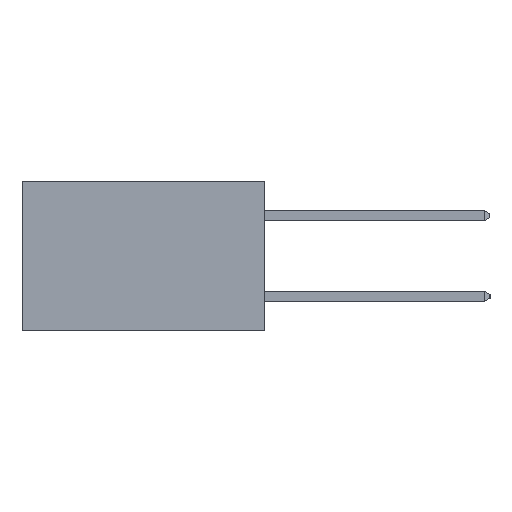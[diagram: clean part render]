
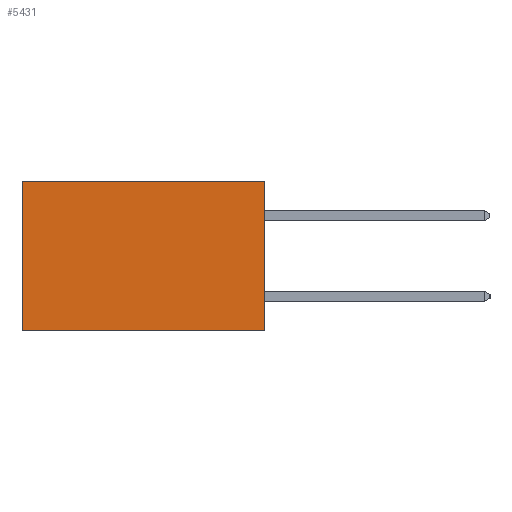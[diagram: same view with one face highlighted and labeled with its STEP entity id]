
A CAD part, left-side view. The second image highlights one B-rep face of the part: STEP entity #5431.
In plain terms, the highlighted planar face has unit normal (-1, 0, 0).
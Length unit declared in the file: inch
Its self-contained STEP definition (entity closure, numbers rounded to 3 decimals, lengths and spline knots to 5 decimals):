
#2610 = VERTEX_POINT ( 'NONE', #9504 ) ;
#2677 = AXIS2_PLACEMENT_3D ( 'NONE', #11544, #11510, #11526 ) ;
#2816 = EDGE_CURVE ( 'NONE', #2610, #10368, #5784, .T. ) ;
#3346 = CARTESIAN_POINT ( 'NONE',  ( 0.2615, 0.6, 0. ) ) ;
#4077 = EDGE_LOOP ( 'NONE', ( #8986, #8988, #9220, #9370 ) ) ;
#4092 = VECTOR ( 'NONE', #6072, 39.37008 ) ;
#4214 = CARTESIAN_POINT ( 'NONE',  ( 0.2615, 0., -0.37 ) ) ;
#4451 = LINE ( 'NONE', #5585, #4092 ) ;
#5192 = VECTOR ( 'NONE', #10935, 39.37008 ) ;
#5406 = VECTOR ( 'NONE', #7824, 39.37008 ) ;
#5431 = ADVANCED_FACE ( 'NONE', ( #13483 ), #11785, .F. ) ;
#5585 = CARTESIAN_POINT ( 'NONE',  ( 0.2615, 0., -0.37 ) ) ;
#5784 = LINE ( 'NONE', #7882, #5406 ) ;
#6072 = DIRECTION ( 'NONE',  ( 0., 1., 0. ) ) ;
#7824 = DIRECTION ( 'NONE',  ( 0., 1., 0. ) ) ;
#7867 = CARTESIAN_POINT ( 'NONE',  ( 0.2615, 0.6, -0.37 ) ) ;
#7882 = CARTESIAN_POINT ( 'NONE',  ( 0.2615, 0., 0. ) ) ;
#8016 = LINE ( 'NONE', #8340, #11032 ) ;
#8129 = DIRECTION ( 'NONE',  ( 0., 0., -1. ) ) ;
#8340 = CARTESIAN_POINT ( 'NONE',  ( 0.2615, 0.6, -0.37 ) ) ;
#8428 = VERTEX_POINT ( 'NONE', #4214 ) ;
#8986 = ORIENTED_EDGE ( 'NONE', *, *, #9615, .T. ) ;
#8988 = ORIENTED_EDGE ( 'NONE', *, *, #13577, .F. ) ;
#9220 = ORIENTED_EDGE ( 'NONE', *, *, #13903, .F. ) ;
#9370 = ORIENTED_EDGE ( 'NONE', *, *, #2816, .T. ) ;
#9504 = CARTESIAN_POINT ( 'NONE',  ( 0.2615, 0., 0. ) ) ;
#9615 = EDGE_CURVE ( 'NONE', #10368, #13516, #8016, .T. ) ;
#10181 = CARTESIAN_POINT ( 'NONE',  ( 0.2615, 0., -0.37 ) ) ;
#10368 = VERTEX_POINT ( 'NONE', #3346 ) ;
#10935 = DIRECTION ( 'NONE',  ( 0., 0., -1. ) ) ;
#11032 = VECTOR ( 'NONE', #8129, 39.37008 ) ;
#11274 = LINE ( 'NONE', #10181, #5192 ) ;
#11510 = DIRECTION ( 'NONE',  ( 1., 0., 0. ) ) ;
#11526 = DIRECTION ( 'NONE',  ( 0., 0., -1. ) ) ;
#11544 = CARTESIAN_POINT ( 'NONE',  ( 0.2615, 0., -0.37 ) ) ;
#11785 = PLANE ( 'NONE',  #2677 ) ;
#13483 = FACE_OUTER_BOUND ( 'NONE', #4077, .T. ) ;
#13516 = VERTEX_POINT ( 'NONE', #7867 ) ;
#13577 = EDGE_CURVE ( 'NONE', #8428, #13516, #4451, .T. ) ;
#13903 = EDGE_CURVE ( 'NONE', #2610, #8428, #11274, .T. ) ;
